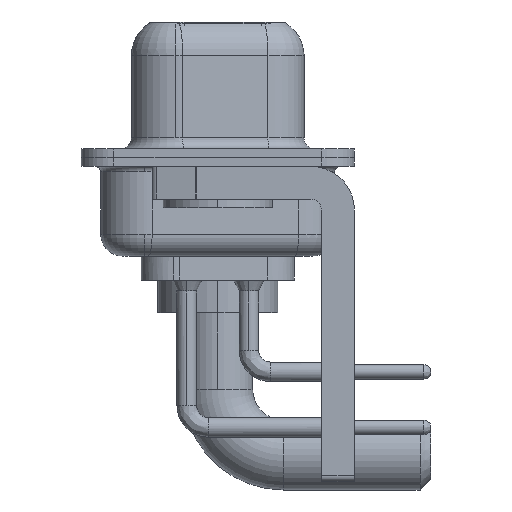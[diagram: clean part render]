
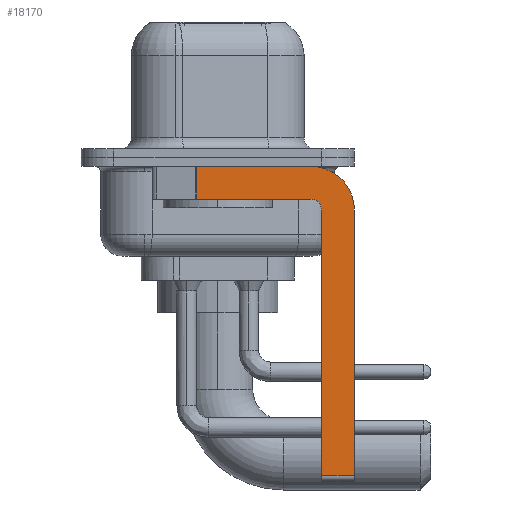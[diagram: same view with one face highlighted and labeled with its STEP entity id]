
A CAD part, left-side view. The second image highlights one B-rep face of the part: STEP entity #18170.
In plain terms, the highlighted planar face has unit normal (-1, 0, 0).
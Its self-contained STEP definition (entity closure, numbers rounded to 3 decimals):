
#97 = VERTEX_POINT ( 'NONE', #15309 ) ;
#447 = CIRCLE ( 'NONE', #7661, 0.5 ) ;
#692 = VERTEX_POINT ( 'NONE', #5545 ) ;
#1339 = VERTEX_POINT ( 'NONE', #13666 ) ;
#1475 = DIRECTION ( 'NONE',  ( 0., 1., 0. ) ) ;
#1650 = CARTESIAN_POINT ( 'NONE',  ( -2.9, 0.978, -0.4 ) ) ;
#1945 = ORIENTED_EDGE ( 'NONE', *, *, #2307, .T. ) ;
#2307 = EDGE_CURVE ( 'NONE', #6994, #1339, #13427, .T. ) ;
#2405 = EDGE_LOOP ( 'NONE', ( #9131, #1945, #13739, #18608, #19084, #2764, #13323, #11363 ) ) ;
#2738 = VERTEX_POINT ( 'NONE', #4234 ) ;
#2764 = ORIENTED_EDGE ( 'NONE', *, *, #5050, .T. ) ;
#3243 = VECTOR ( 'NONE', #18010, 1000. ) ;
#3805 = CARTESIAN_POINT ( 'NONE',  ( -2.9, -4.25, -2.4 ) ) ;
#4223 = CARTESIAN_POINT ( 'NONE',  ( -2.9, -4.25, -1.9 ) ) ;
#4234 = CARTESIAN_POINT ( 'NONE',  ( -2.9, -4.75, -14.55 ) ) ;
#5050 = EDGE_CURVE ( 'NONE', #2738, #10821, #6007, .T. ) ;
#5196 = DIRECTION ( 'NONE',  ( 0., 0., 1. ) ) ;
#5330 = EDGE_CURVE ( 'NONE', #97, #16787, #447, .T. ) ;
#5537 = VECTOR ( 'NONE', #14131, 1000. ) ;
#5545 = CARTESIAN_POINT ( 'NONE',  ( -2.9, -6.25, -2.4 ) ) ;
#6007 = LINE ( 'NONE', #10356, #3243 ) ;
#6027 = CARTESIAN_POINT ( 'NONE',  ( -2.9, 0.978, -1.9 ) ) ;
#6126 = DIRECTION ( 'NONE',  ( 0., 0., -1. ) ) ;
#6994 = VERTEX_POINT ( 'NONE', #1650 ) ;
#7661 = AXIS2_PLACEMENT_3D ( 'NONE', #19160, #15921, #16020 ) ;
#7817 = CARTESIAN_POINT ( 'NONE',  ( -2.9, -6.25, -2.4 ) ) ;
#8802 = CARTESIAN_POINT ( 'NONE',  ( -2.9, 3., -0.4 ) ) ;
#9131 = ORIENTED_EDGE ( 'NONE', *, *, #11707, .F. ) ;
#9506 = LINE ( 'NONE', #7817, #5537 ) ;
#10095 = VECTOR ( 'NONE', #6126, 1000. ) ;
#10154 = LINE ( 'NONE', #4223, #10806 ) ;
#10293 = DIRECTION ( 'NONE',  ( 0., -1., 0. ) ) ;
#10356 = CARTESIAN_POINT ( 'NONE',  ( -2.9, -4.25, -14.55 ) ) ;
#10601 = AXIS2_PLACEMENT_3D ( 'NONE', #3805, #19073, #17307 ) ;
#10806 = VECTOR ( 'NONE', #1475, 1000. ) ;
#10821 = VERTEX_POINT ( 'NONE', #13490 ) ;
#11363 = ORIENTED_EDGE ( 'NONE', *, *, #16867, .F. ) ;
#11707 = EDGE_CURVE ( 'NONE', #6994, #15940, #16192, .T. ) ;
#11820 = AXIS2_PLACEMENT_3D ( 'NONE', #14352, #15822, #15923 ) ;
#12684 = LINE ( 'NONE', #14057, #15843 ) ;
#13323 = ORIENTED_EDGE ( 'NONE', *, *, #18437, .F. ) ;
#13427 = LINE ( 'NONE', #6027, #10095 ) ;
#13490 = CARTESIAN_POINT ( 'NONE',  ( -2.9, -6.25, -14.55 ) ) ;
#13666 = CARTESIAN_POINT ( 'NONE',  ( -2.9, 0.978, -1.9 ) ) ;
#13739 = ORIENTED_EDGE ( 'NONE', *, *, #14541, .F. ) ;
#14057 = CARTESIAN_POINT ( 'NONE',  ( -2.9, -4.75, -14.8 ) ) ;
#14131 = DIRECTION ( 'NONE',  ( 0., 0., -1. ) ) ;
#14352 = CARTESIAN_POINT ( 'NONE',  ( -2.9, -4.25, -2.4 ) ) ;
#14541 = EDGE_CURVE ( 'NONE', #16787, #1339, #10154, .T. ) ;
#14925 = EDGE_CURVE ( 'NONE', #2738, #97, #12684, .T. ) ;
#15079 = VECTOR ( 'NONE', #10293, 1000. ) ;
#15309 = CARTESIAN_POINT ( 'NONE',  ( -2.9, -4.75, -2.4 ) ) ;
#15822 = DIRECTION ( 'NONE',  ( 1., 0., 0. ) ) ;
#15843 = VECTOR ( 'NONE', #5196, 1000. ) ;
#15921 = DIRECTION ( 'NONE',  ( -1., 0., 0. ) ) ;
#15923 = DIRECTION ( 'NONE',  ( 0., 0., -1. ) ) ;
#15940 = VERTEX_POINT ( 'NONE', #16591 ) ;
#16020 = DIRECTION ( 'NONE',  ( 0., 0., 1. ) ) ;
#16118 = FACE_OUTER_BOUND ( 'NONE', #2405, .T. ) ;
#16192 = LINE ( 'NONE', #8802, #15079 ) ;
#16591 = CARTESIAN_POINT ( 'NONE',  ( -2.9, -4.25, -0.4 ) ) ;
#16787 = VERTEX_POINT ( 'NONE', #18275 ) ;
#16867 = EDGE_CURVE ( 'NONE', #15940, #692, #19045, .T. ) ;
#17307 = DIRECTION ( 'NONE',  ( 0., 0., -1. ) ) ;
#18010 = DIRECTION ( 'NONE',  ( 0., -1., 0. ) ) ;
#18170 = ADVANCED_FACE ( 'NONE', ( #16118 ), #19164, .F. ) ;
#18275 = CARTESIAN_POINT ( 'NONE',  ( -2.9, -4.25, -1.9 ) ) ;
#18437 = EDGE_CURVE ( 'NONE', #692, #10821, #9506, .T. ) ;
#18608 = ORIENTED_EDGE ( 'NONE', *, *, #5330, .F. ) ;
#19045 = CIRCLE ( 'NONE', #11820, 2. ) ;
#19073 = DIRECTION ( 'NONE',  ( 1., 0., 0. ) ) ;
#19084 = ORIENTED_EDGE ( 'NONE', *, *, #14925, .F. ) ;
#19160 = CARTESIAN_POINT ( 'NONE',  ( -2.9, -4.25, -2.4 ) ) ;
#19164 = PLANE ( 'NONE',  #10601 ) ;
